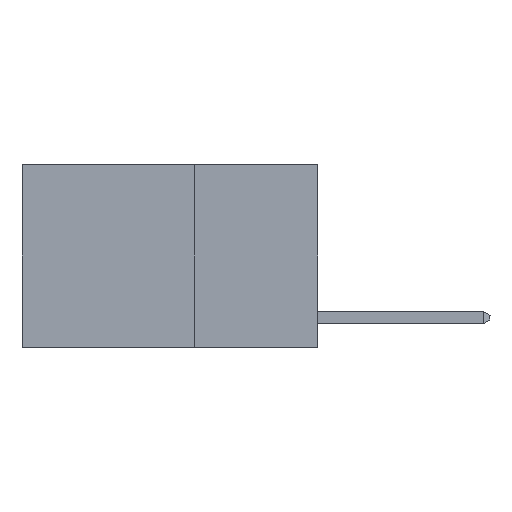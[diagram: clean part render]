
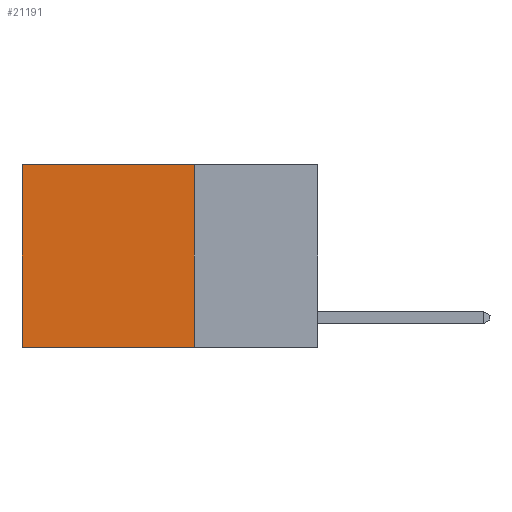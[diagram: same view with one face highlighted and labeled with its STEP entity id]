
A CAD part, left-side view. The second image highlights one B-rep face of the part: STEP entity #21191.
In plain terms, the highlighted planar face has unit normal (-1, 0, 0).
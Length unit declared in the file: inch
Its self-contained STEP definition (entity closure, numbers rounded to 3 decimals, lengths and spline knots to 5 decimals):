
#418 = FACE_OUTER_BOUND ( 'NONE', #912, .T. ) ;
#703 = DIRECTION ( 'NONE',  ( 0., 0., -1. ) ) ;
#912 = EDGE_LOOP ( 'NONE', ( #1302, #2636, #17260, #3734 ) ) ;
#1143 = VECTOR ( 'NONE', #4600, 39.37008 ) ;
#1302 = ORIENTED_EDGE ( 'NONE', *, *, #21034, .T. ) ;
#1640 = CARTESIAN_POINT ( 'NONE',  ( 0.2625, 0.25, 0. ) ) ;
#1734 = DIRECTION ( 'NONE',  ( 0., 0., -1. ) ) ;
#2636 = ORIENTED_EDGE ( 'NONE', *, *, #2876, .F. ) ;
#2876 = EDGE_CURVE ( 'NONE', #18749, #19624, #18639, .T. ) ;
#3303 = DIRECTION ( 'NONE',  ( 0., 0., -1. ) ) ;
#3362 = CARTESIAN_POINT ( 'NONE',  ( 0.2625, 0.25, -0.37 ) ) ;
#3734 = ORIENTED_EDGE ( 'NONE', *, *, #15322, .T. ) ;
#4590 = VECTOR ( 'NONE', #703, 39.37008 ) ;
#4600 = DIRECTION ( 'NONE',  ( 0., 1., 0. ) ) ;
#6672 = LINE ( 'NONE', #16737, #1143 ) ;
#10904 = CARTESIAN_POINT ( 'NONE',  ( 0.2625, 0.25, 0. ) ) ;
#11931 = EDGE_CURVE ( 'NONE', #21087, #18749, #20781, .T. ) ;
#12578 = VECTOR ( 'NONE', #17567, 39.37008 ) ;
#13951 = DIRECTION ( 'NONE',  ( 1., 0., 0. ) ) ;
#14496 = LINE ( 'NONE', #15474, #20554 ) ;
#14738 = CARTESIAN_POINT ( 'NONE',  ( 0.2625, 0.6, -0.37 ) ) ;
#15322 = EDGE_CURVE ( 'NONE', #21087, #18149, #6672, .T. ) ;
#15474 = CARTESIAN_POINT ( 'NONE',  ( 0.2625, 0.6, 0. ) ) ;
#16737 = CARTESIAN_POINT ( 'NONE',  ( 0.2625, 0.25, 0. ) ) ;
#17260 = ORIENTED_EDGE ( 'NONE', *, *, #11931, .F. ) ;
#17567 = DIRECTION ( 'NONE',  ( 0., 1., 0. ) ) ;
#17609 = CARTESIAN_POINT ( 'NONE',  ( 0.2625, 0.25, 0. ) ) ;
#18149 = VERTEX_POINT ( 'NONE', #26050 ) ;
#18639 = LINE ( 'NONE', #3362, #12578 ) ;
#18749 = VERTEX_POINT ( 'NONE', #25833 ) ;
#19624 = VERTEX_POINT ( 'NONE', #14738 ) ;
#20554 = VECTOR ( 'NONE', #3303, 39.37008 ) ;
#20781 = LINE ( 'NONE', #10904, #4590 ) ;
#21034 = EDGE_CURVE ( 'NONE', #18149, #19624, #14496, .T. ) ;
#21087 = VERTEX_POINT ( 'NONE', #17609 ) ;
#21191 = ADVANCED_FACE ( 'NONE', ( #418 ), #22079, .F. ) ;
#22079 = PLANE ( 'NONE',  #22830 ) ;
#22830 = AXIS2_PLACEMENT_3D ( 'NONE', #1640, #13951, #1734 ) ;
#25833 = CARTESIAN_POINT ( 'NONE',  ( 0.2625, 0.25, -0.37 ) ) ;
#26050 = CARTESIAN_POINT ( 'NONE',  ( 0.2625, 0.6, 0. ) ) ;
